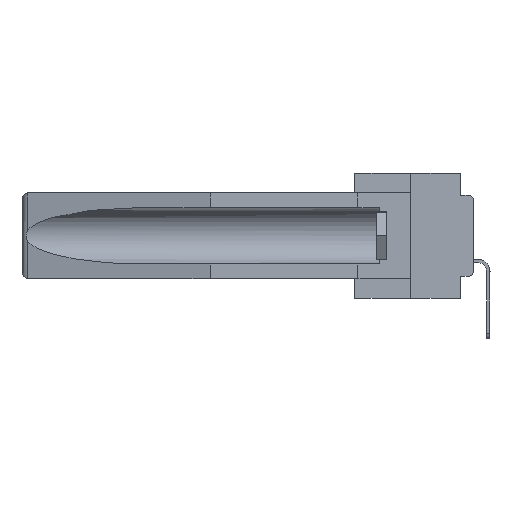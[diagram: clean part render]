
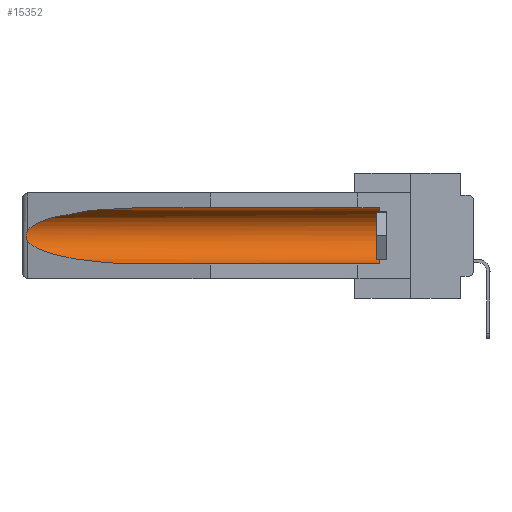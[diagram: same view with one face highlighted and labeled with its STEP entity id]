
A CAD part, left-side view. The second image highlights one B-rep face of the part: STEP entity #15352.
In plain terms, the highlighted cylindrical face has radius 2.857 mm (diameter 5.715 mm), a partial arc.
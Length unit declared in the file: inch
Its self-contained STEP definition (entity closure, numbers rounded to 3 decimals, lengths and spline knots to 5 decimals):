
#497 = CARTESIAN_POINT ( 'NONE',  ( 0.2673, 1.5327, -0.16383 ) ) ;
#2042 = DIRECTION ( 'NONE',  ( 0., -1., 0. ) ) ;
#2329 = ORIENTED_EDGE ( 'NONE', *, *, #30182, .T. ) ;
#2525 = CARTESIAN_POINT ( 'NONE',  ( 0.155, -0.30754, -0.1715 ) ) ;
#3099 = FACE_OUTER_BOUND ( 'NONE', #33494, .T. ) ;
#3238 = DIRECTION ( 'NONE',  ( 0., 1., 0. ) ) ;
#3542 = EDGE_CURVE ( 'NONE', #35561, #26280, #17192, .T. ) ;
#4313 = CARTESIAN_POINT ( 'NONE',  ( 0.26597, 1.5296, -0.19026 ) ) ;
#5242 = ORIENTED_EDGE ( 'NONE', *, *, #28586, .T. ) ;
#5852 = AXIS2_PLACEMENT_3D ( 'NONE', #19254, #2042, #27890 ) ;
#6426 = B_SPLINE_CURVE_WITH_KNOTS ( 'NONE', 3,
 ( #23672, #15030, #32460, #497, #35515, #12169, #33412, #36277, #4313, #15778 ),
 .UNSPECIFIED., .F., .F.,
 ( 4, 2, 2, 2, 4 ),
 ( 0., 0.00029, 0.00058, 0.00087, 0.00117 ),
 .UNSPECIFIED. ) ;
#6574 = CARTESIAN_POINT ( 'NONE',  ( 0.26537, 1.52718, -0.19328 ) ) ;
#8839 = DIRECTION ( 'NONE',  ( 0., 0., 1. ) ) ;
#8953 = CARTESIAN_POINT ( 'NONE',  ( 0.26537, 1.52718, -0.14972 ) ) ;
#9260 = VECTOR ( 'NONE', #26819, 39.37008 ) ;
#9865 = AXIS2_PLACEMENT_3D ( 'NONE', #2525, #26437, #8839 ) ;
#10380 = ORIENTED_EDGE ( 'NONE', *, *, #3542, .F. ) ;
#10950 = CARTESIAN_POINT ( 'NONE',  ( 0.155, 1.07973, -0.059 ) ) ;
#11332 = ORIENTED_EDGE ( 'NONE', *, *, #36950, .T. ) ;
#11393 = CARTESIAN_POINT ( 'NONE',  ( 0.26537, 1.52718, -0.19328 ) ) ;
#11404 = CARTESIAN_POINT ( 'NONE',  ( 0.25451, 1.48313, -0.09465 ) ) ;
#11926 = ORIENTED_EDGE ( 'NONE', *, *, #27477, .T. ) ;
#12169 = CARTESIAN_POINT ( 'NONE',  ( 0.2675, 1.53308, -0.17534 ) ) ;
#13788 = CIRCLE ( 'NONE', #5852, 0.1125 ) ;
#15030 = CARTESIAN_POINT ( 'NONE',  ( 0.26597, 1.52961, -0.15275 ) ) ;
#15124 = CARTESIAN_POINT ( 'NONE',  ( 0.155, -0.30754, -0.059 ) ) ;
#15352 = ADVANCED_FACE ( 'NONE', ( #3099 ), #26248, .F. ) ;
#15599 = EDGE_CURVE ( 'NONE', #32537, #26157, #18000, .T. ) ;
#15778 = CARTESIAN_POINT ( 'NONE',  ( 0.26537, 1.52718, -0.19328 ) ) ;
#16737 = ORIENTED_EDGE ( 'NONE', *, *, #15599, .T. ) ;
#17192 = LINE ( 'NONE', #28876, #37418 ) ;
#17459 = VERTEX_POINT ( 'NONE', #8953 ) ;
#18000 = LINE ( 'NONE', #15124, #9260 ) ;
#18602 = CARTESIAN_POINT ( 'NONE',  ( 0.21114, 1.30732, -0.284 ) ) ;
#19254 = CARTESIAN_POINT ( 'NONE',  ( 0.155, 0.126, -0.1715 ) ) ;
#20838 = VERTEX_POINT ( 'NONE', #11393 ) ;
#23672 = CARTESIAN_POINT ( 'NONE',  ( 0.26537, 1.52718, -0.14972 ) ) ;
#25378 = CARTESIAN_POINT ( 'NONE',  ( 0.155, 1.07973, -0.059 ) ) ;
#25702 = CARTESIAN_POINT ( 'NONE',  ( 0.155, 0.126, -0.284 ) ) ;
#25936 = CARTESIAN_POINT ( 'NONE',  ( 0.21114, 1.30732, -0.059 ) ) ;
#26157 = VERTEX_POINT ( 'NONE', #10950 ) ;
#26248 = CYLINDRICAL_SURFACE ( 'NONE', #9865, 0.1125 ) ;
#26280 = VERTEX_POINT ( 'NONE', #37731 ) ;
#26437 = DIRECTION ( 'NONE',  ( 0., 1., 0. ) ) ;
#26819 = DIRECTION ( 'NONE',  ( 0., 1., 0. ) ) ;
#27413 = CARTESIAN_POINT ( 'NONE',  ( 0.155, 1.07973, -0.284 ) ) ;
#27477 = EDGE_CURVE ( 'NONE', #26157, #17459, #32965, .T. ) ;
#27890 = DIRECTION ( 'NONE',  ( 0., 0., 1. ) ) ;
#28586 = EDGE_CURVE ( 'NONE', #35561, #32537, #13788, .T. ) ;
#28876 = CARTESIAN_POINT ( 'NONE',  ( 0.155, -0.30754, -0.284 ) ) ;
#29908 = CARTESIAN_POINT ( 'NONE',  ( 0.25451, 1.48313, -0.24835 ) ) ;
#30182 = EDGE_CURVE ( 'NONE', #17459, #20838, #6426, .T. ) ;
#32460 = CARTESIAN_POINT ( 'NONE',  ( 0.26654, 1.53092, -0.15636 ) ) ;
#32537 = VERTEX_POINT ( 'NONE', #33289 ) ;
#32965 =( BOUNDED_CURVE ( )  B_SPLINE_CURVE ( 3, ( #25378, #25936, #11404, #34764 ),
 .UNSPECIFIED., .F., .T. ) 
 B_SPLINE_CURVE_WITH_KNOTS ( ( 4, 4 ),
 ( 4.71239, 6.08839 ),
 .UNSPECIFIED. ) 
 CURVE ( )  GEOMETRIC_REPRESENTATION_ITEM ( )  RATIONAL_B_SPLINE_CURVE ( ( 1., 0.848, 0.848, 1. ) ) 
 REPRESENTATION_ITEM ( '' )  );
#33289 = CARTESIAN_POINT ( 'NONE',  ( 0.155, 0.126, -0.059 ) ) ;
#33412 = CARTESIAN_POINT ( 'NONE',  ( 0.2673, 1.53269, -0.17917 ) ) ;
#33494 = EDGE_LOOP ( 'NONE', ( #11926, #2329, #11332, #10380, #5242, #16737 ) ) ;
#34764 = CARTESIAN_POINT ( 'NONE',  ( 0.26537, 1.52718, -0.14972 ) ) ;
#35515 = CARTESIAN_POINT ( 'NONE',  ( 0.2675, 1.53308, -0.16763 ) ) ;
#35561 = VERTEX_POINT ( 'NONE', #25702 ) ;
#36277 = CARTESIAN_POINT ( 'NONE',  ( 0.26655, 1.53094, -0.18657 ) ) ;
#36880 =( BOUNDED_CURVE ( )  B_SPLINE_CURVE ( 3, ( #6574, #29908, #18602, #27413 ),
 .UNSPECIFIED., .F., .T. ) 
 B_SPLINE_CURVE_WITH_KNOTS ( ( 4, 4 ),
 ( 0.1948, 1.5708 ),
 .UNSPECIFIED. ) 
 CURVE ( )  GEOMETRIC_REPRESENTATION_ITEM ( )  RATIONAL_B_SPLINE_CURVE ( ( 1., 0.848, 0.848, 1. ) ) 
 REPRESENTATION_ITEM ( '' )  );
#36950 = EDGE_CURVE ( 'NONE', #20838, #26280, #36880, .T. ) ;
#37418 = VECTOR ( 'NONE', #3238, 39.37008 ) ;
#37731 = CARTESIAN_POINT ( 'NONE',  ( 0.155, 1.07973, -0.284 ) ) ;
